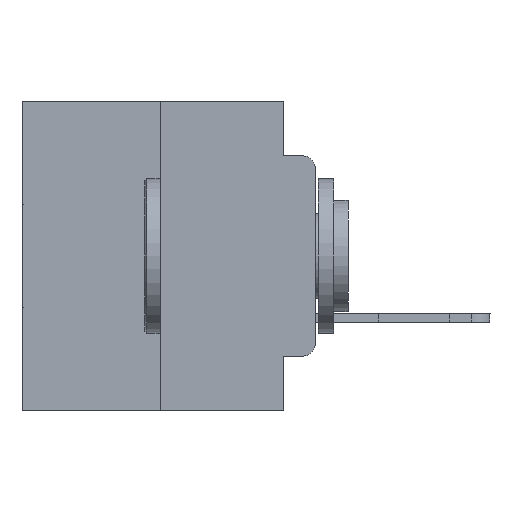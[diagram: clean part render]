
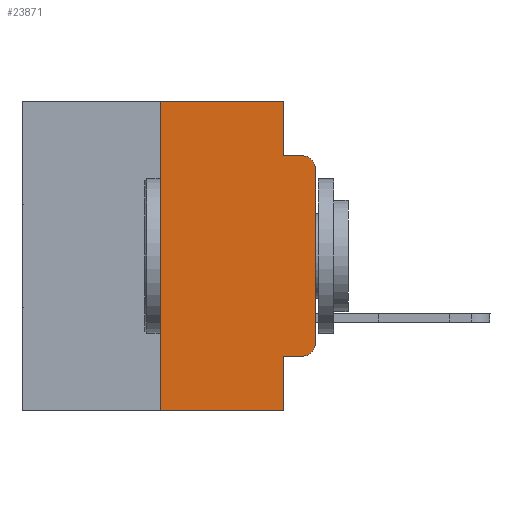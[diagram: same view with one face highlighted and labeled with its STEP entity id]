
A CAD part, left-side view. The second image highlights one B-rep face of the part: STEP entity #23871.
In plain terms, the highlighted planar face has unit normal (-1, 0, 0).
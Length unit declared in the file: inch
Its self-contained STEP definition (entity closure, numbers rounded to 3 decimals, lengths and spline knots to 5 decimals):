
#198 = ORIENTED_EDGE ( 'NONE', *, *, #23218, .T. ) ;
#717 = CARTESIAN_POINT ( 'NONE',  ( 0., 0.051, -0.0885 ) ) ;
#882 = ORIENTED_EDGE ( 'NONE', *, *, #14870, .T. ) ;
#1290 = CARTESIAN_POINT ( 'NONE',  ( 0., 0.25, 0. ) ) ;
#1458 = ORIENTED_EDGE ( 'NONE', *, *, #15533, .F. ) ;
#1721 = CARTESIAN_POINT ( 'NONE',  ( 0., 0.02, -0.3915 ) ) ;
#1831 = ORIENTED_EDGE ( 'NONE', *, *, #17707, .F. ) ;
#1985 = CARTESIAN_POINT ( 'NONE',  ( 0., 0.25, -0.5 ) ) ;
#2529 = CARTESIAN_POINT ( 'NONE',  ( 0., 0.051, 0. ) ) ;
#2757 = DIRECTION ( 'NONE',  ( 0., -1., 0. ) ) ;
#2870 = VERTEX_POINT ( 'NONE', #8924 ) ;
#2958 = VERTEX_POINT ( 'NONE', #717 ) ;
#3041 = VERTEX_POINT ( 'NONE', #27662 ) ;
#3496 = EDGE_CURVE ( 'NONE', #8333, #18244, #24618, .T. ) ;
#3807 = VERTEX_POINT ( 'NONE', #22119 ) ;
#3856 = VECTOR ( 'NONE', #26889, 39.37008 ) ;
#4215 = ORIENTED_EDGE ( 'NONE', *, *, #12457, .T. ) ;
#5530 = AXIS2_PLACEMENT_3D ( 'NONE', #20796, #16394, #25320 ) ;
#6035 = CIRCLE ( 'NONE', #26636, 0.02 ) ;
#6845 = CARTESIAN_POINT ( 'NONE',  ( 0., 0.051, 0. ) ) ;
#7496 = LINE ( 'NONE', #27122, #13729 ) ;
#7970 = ORIENTED_EDGE ( 'NONE', *, *, #15174, .F. ) ;
#8333 = VERTEX_POINT ( 'NONE', #15223 ) ;
#8465 = DIRECTION ( 'NONE',  ( 0., 0., -1. ) ) ;
#8581 = VECTOR ( 'NONE', #2757, 39.37008 ) ;
#8924 = CARTESIAN_POINT ( 'NONE',  ( 0., 0., -0.3915 ) ) ;
#9259 = DIRECTION ( 'NONE',  ( 0., -1., 0. ) ) ;
#9379 = VERTEX_POINT ( 'NONE', #2529 ) ;
#10264 = DIRECTION ( 'NONE',  ( 0., 0., -1. ) ) ;
#10407 = ORIENTED_EDGE ( 'NONE', *, *, #22720, .T. ) ;
#11428 = CARTESIAN_POINT ( 'NONE',  ( 0., 0.051, -0.0885 ) ) ;
#11577 = PLANE ( 'NONE',  #5530 ) ;
#11622 = LINE ( 'NONE', #18191, #11802 ) ;
#11802 = VECTOR ( 'NONE', #9259, 39.37008 ) ;
#11874 = FACE_OUTER_BOUND ( 'NONE', #25365, .T. ) ;
#12457 = EDGE_CURVE ( 'NONE', #8333, #3807, #11622, .T. ) ;
#13729 = VECTOR ( 'NONE', #16431, 39.37008 ) ;
#13986 = LINE ( 'NONE', #24812, #26448 ) ;
#14673 = DIRECTION ( 'NONE',  ( -1., 0., 0. ) ) ;
#14719 = ORIENTED_EDGE ( 'NONE', *, *, #3496, .F. ) ;
#14810 = VERTEX_POINT ( 'NONE', #1985 ) ;
#14870 = EDGE_CURVE ( 'NONE', #14810, #18244, #17662, .T. ) ;
#15174 = EDGE_CURVE ( 'NONE', #23070, #9379, #7496, .T. ) ;
#15223 = CARTESIAN_POINT ( 'NONE',  ( 0., 0.051, -0.4115 ) ) ;
#15533 = EDGE_CURVE ( 'NONE', #2958, #3041, #27083, .T. ) ;
#15746 = DIRECTION ( 'NONE',  ( 0., 0., 1. ) ) ;
#16079 = ORIENTED_EDGE ( 'NONE', *, *, #25449, .F. ) ;
#16394 = DIRECTION ( 'NONE',  ( 1., 0., 0. ) ) ;
#16431 = DIRECTION ( 'NONE',  ( 0., -1., 0. ) ) ;
#17662 = LINE ( 'NONE', #17809, #3856 ) ;
#17707 = EDGE_CURVE ( 'NONE', #14810, #23070, #13986, .T. ) ;
#17809 = CARTESIAN_POINT ( 'NONE',  ( 0., 0.473, -0.5 ) ) ;
#18191 = CARTESIAN_POINT ( 'NONE',  ( 0., 0.051, -0.4115 ) ) ;
#18244 = VERTEX_POINT ( 'NONE', #19333 ) ;
#19170 = EDGE_CURVE ( 'NONE', #2870, #19430, #21184, .T. ) ;
#19333 = CARTESIAN_POINT ( 'NONE',  ( 0., 0.051, -0.5 ) ) ;
#19430 = VERTEX_POINT ( 'NONE', #20416 ) ;
#20416 = CARTESIAN_POINT ( 'NONE',  ( 0., 0., -0.1085 ) ) ;
#20796 = CARTESIAN_POINT ( 'NONE',  ( 0., 0.473, 0. ) ) ;
#21184 = LINE ( 'NONE', #28196, #25967 ) ;
#22097 = LINE ( 'NONE', #6845, #22421 ) ;
#22119 = CARTESIAN_POINT ( 'NONE',  ( 0., 0.02, -0.4115 ) ) ;
#22421 = VECTOR ( 'NONE', #26622, 39.37008 ) ;
#22579 = DIRECTION ( 'NONE',  ( 0., 0., -1. ) ) ;
#22720 = EDGE_CURVE ( 'NONE', #19430, #3041, #25214, .T. ) ;
#23070 = VERTEX_POINT ( 'NONE', #1290 ) ;
#23218 = EDGE_CURVE ( 'NONE', #3807, #2870, #6035, .T. ) ;
#23871 = ADVANCED_FACE ( 'NONE', ( #11874 ), #11577, .F. ) ;
#24618 = LINE ( 'NONE', #27117, #25082 ) ;
#24812 = CARTESIAN_POINT ( 'NONE',  ( 0., 0.25, 0. ) ) ;
#25082 = VECTOR ( 'NONE', #22579, 39.37008 ) ;
#25214 = CIRCLE ( 'NONE', #28962, 0.02 ) ;
#25320 = DIRECTION ( 'NONE',  ( 0., 0., -1. ) ) ;
#25365 = EDGE_LOOP ( 'NONE', ( #28139, #10407, #1458, #16079, #7970, #1831, #882, #14719, #4215, #198 ) ) ;
#25449 = EDGE_CURVE ( 'NONE', #9379, #2958, #22097, .T. ) ;
#25785 = CARTESIAN_POINT ( 'NONE',  ( 0., 0.02, -0.1085 ) ) ;
#25967 = VECTOR ( 'NONE', #27905, 39.37008 ) ;
#26448 = VECTOR ( 'NONE', #15746, 39.37008 ) ;
#26622 = DIRECTION ( 'NONE',  ( 0., 0., -1. ) ) ;
#26636 = AXIS2_PLACEMENT_3D ( 'NONE', #1721, #28386, #8465 ) ;
#26889 = DIRECTION ( 'NONE',  ( 0., -1., 0. ) ) ;
#27083 = LINE ( 'NONE', #11428, #8581 ) ;
#27117 = CARTESIAN_POINT ( 'NONE',  ( 0., 0.051, 0. ) ) ;
#27122 = CARTESIAN_POINT ( 'NONE',  ( 0., 0.473, 0. ) ) ;
#27662 = CARTESIAN_POINT ( 'NONE',  ( 0., 0.02, -0.0885 ) ) ;
#27905 = DIRECTION ( 'NONE',  ( 0., 0., 1. ) ) ;
#28139 = ORIENTED_EDGE ( 'NONE', *, *, #19170, .T. ) ;
#28196 = CARTESIAN_POINT ( 'NONE',  ( 0., 0., 0. ) ) ;
#28386 = DIRECTION ( 'NONE',  ( -1., 0., 0. ) ) ;
#28962 = AXIS2_PLACEMENT_3D ( 'NONE', #25785, #14673, #10264 ) ;
